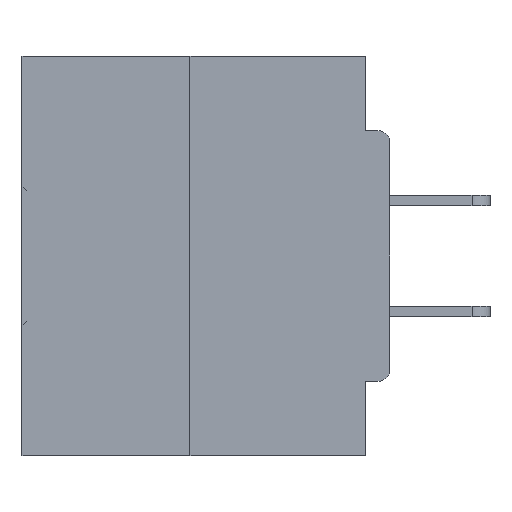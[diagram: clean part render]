
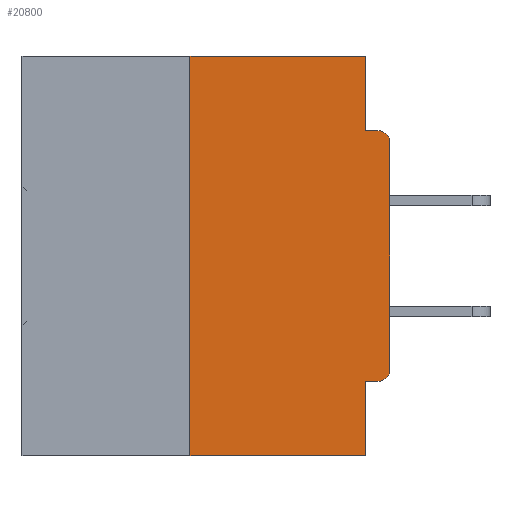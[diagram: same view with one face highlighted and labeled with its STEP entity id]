
A CAD part, left-side view. The second image highlights one B-rep face of the part: STEP entity #20800.
In plain terms, the highlighted planar face has unit normal (-1, 0, 0).
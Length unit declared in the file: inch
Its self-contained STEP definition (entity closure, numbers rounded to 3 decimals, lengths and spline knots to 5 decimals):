
#167 = VERTEX_POINT ( 'NONE', #30336 ) ;
#1050 = CARTESIAN_POINT ( 'NONE',  ( 0., 0.46, 0. ) ) ;
#2170 = VECTOR ( 'NONE', #42823, 39.37008 ) ;
#2192 = VECTOR ( 'NONE', #34902, 39.37008 ) ;
#2277 = LINE ( 'NONE', #28253, #13767 ) ;
#2855 = CARTESIAN_POINT ( 'NONE',  ( 0., 0.015, -0.0935 ) ) ;
#2877 = DIRECTION ( 'NONE',  ( -1., 0., 0. ) ) ;
#3250 = LINE ( 'NONE', #1050, #27446 ) ;
#4359 = CARTESIAN_POINT ( 'NONE',  ( 0., 0.031, 0. ) ) ;
#4479 = DIRECTION ( 'NONE',  ( 0., 0., 1. ) ) ;
#4711 = CARTESIAN_POINT ( 'NONE',  ( 0., 0.031, -0.5 ) ) ;
#4830 = AXIS2_PLACEMENT_3D ( 'NONE', #22929, #5568, #40693 ) ;
#5480 = VERTEX_POINT ( 'NONE', #2855 ) ;
#5568 = DIRECTION ( 'NONE',  ( 1., 0., 0. ) ) ;
#5937 = CARTESIAN_POINT ( 'NONE',  ( 0., 0.015, -0.3915 ) ) ;
#6063 = CARTESIAN_POINT ( 'NONE',  ( 0., 0.25, 0. ) ) ;
#6618 = CARTESIAN_POINT ( 'NONE',  ( 0., 0., -0.1085 ) ) ;
#7210 = DIRECTION ( 'NONE',  ( 0., -1., 0. ) ) ;
#8270 = EDGE_CURVE ( 'NONE', #15106, #21695, #12158, .T. ) ;
#8467 = CARTESIAN_POINT ( 'NONE',  ( 0., 0., -0.4065 ) ) ;
#8943 = EDGE_CURVE ( 'NONE', #15106, #167, #39722, .T. ) ;
#8954 = DIRECTION ( 'NONE',  ( -1., 0., 0. ) ) ;
#9755 = FACE_OUTER_BOUND ( 'NONE', #16132, .T. ) ;
#9790 = ORIENTED_EDGE ( 'NONE', *, *, #42804, .F. ) ;
#9899 = CARTESIAN_POINT ( 'NONE',  ( 0., 0.031, -0.4065 ) ) ;
#10273 = EDGE_CURVE ( 'NONE', #17444, #37389, #21950, .T. ) ;
#11295 = DIRECTION ( 'NONE',  ( 0., 0., -1. ) ) ;
#12158 = LINE ( 'NONE', #8467, #38126 ) ;
#12465 = PLANE ( 'NONE',  #4830 ) ;
#13767 = VECTOR ( 'NONE', #7210, 39.37008 ) ;
#13922 = ORIENTED_EDGE ( 'NONE', *, *, #30022, .T. ) ;
#14165 = CIRCLE ( 'NONE', #31103, 0.015 ) ;
#14408 = ORIENTED_EDGE ( 'NONE', *, *, #20055, .F. ) ;
#15106 = VERTEX_POINT ( 'NONE', #30540 ) ;
#16132 = EDGE_LOOP ( 'NONE', ( #14408, #29965, #29493, #41992, #29575, #18487, #26755, #13922, #43258, #9790 ) ) ;
#16295 = LINE ( 'NONE', #6063, #39518 ) ;
#16610 = DIRECTION ( 'NONE',  ( 0., 0., 1. ) ) ;
#17444 = VERTEX_POINT ( 'NONE', #32879 ) ;
#17700 = AXIS2_PLACEMENT_3D ( 'NONE', #5937, #2877, #38313 ) ;
#17887 = VERTEX_POINT ( 'NONE', #24301 ) ;
#18487 = ORIENTED_EDGE ( 'NONE', *, *, #8943, .T. ) ;
#18583 = EDGE_CURVE ( 'NONE', #17887, #5480, #2277, .T. ) ;
#19235 = LINE ( 'NONE', #28235, #2192 ) ;
#20055 = EDGE_CURVE ( 'NONE', #34988, #33807, #3250, .T. ) ;
#20800 = ADVANCED_FACE ( 'NONE', ( #9755 ), #12465, .F. ) ;
#21695 = VERTEX_POINT ( 'NONE', #9899 ) ;
#21950 = LINE ( 'NONE', #24924, #2170 ) ;
#22608 = EDGE_CURVE ( 'NONE', #167, #43945, #30040, .T. ) ;
#22929 = CARTESIAN_POINT ( 'NONE',  ( 0., 0.46, 0. ) ) ;
#23532 = CARTESIAN_POINT ( 'NONE',  ( 0., 0.25, 0. ) ) ;
#24166 = VECTOR ( 'NONE', #11295, 39.37008 ) ;
#24301 = CARTESIAN_POINT ( 'NONE',  ( 0., 0.031, -0.0935 ) ) ;
#24924 = CARTESIAN_POINT ( 'NONE',  ( 0., 0.46, -0.5 ) ) ;
#26755 = ORIENTED_EDGE ( 'NONE', *, *, #22608, .T. ) ;
#27446 = VECTOR ( 'NONE', #33836, 39.37008 ) ;
#28235 = CARTESIAN_POINT ( 'NONE',  ( 0., 0.031, -0.5 ) ) ;
#28253 = CARTESIAN_POINT ( 'NONE',  ( 0., 0., -0.0935 ) ) ;
#29493 = ORIENTED_EDGE ( 'NONE', *, *, #10273, .T. ) ;
#29575 = ORIENTED_EDGE ( 'NONE', *, *, #8270, .F. ) ;
#29883 = CARTESIAN_POINT ( 'NONE',  ( 0., 0.015, -0.1085 ) ) ;
#29965 = ORIENTED_EDGE ( 'NONE', *, *, #37685, .F. ) ;
#30022 = EDGE_CURVE ( 'NONE', #43945, #5480, #14165, .T. ) ;
#30040 = LINE ( 'NONE', #40351, #44885 ) ;
#30336 = CARTESIAN_POINT ( 'NONE',  ( 0., 0., -0.3915 ) ) ;
#30540 = CARTESIAN_POINT ( 'NONE',  ( 0., 0.015, -0.4065 ) ) ;
#31103 = AXIS2_PLACEMENT_3D ( 'NONE', #29883, #8954, #44315 ) ;
#32312 = CARTESIAN_POINT ( 'NONE',  ( 0., 0.031, 0. ) ) ;
#32879 = CARTESIAN_POINT ( 'NONE',  ( 0., 0.25, -0.5 ) ) ;
#33601 = LINE ( 'NONE', #32312, #24166 ) ;
#33807 = VERTEX_POINT ( 'NONE', #4359 ) ;
#33836 = DIRECTION ( 'NONE',  ( 0., -1., 0. ) ) ;
#34902 = DIRECTION ( 'NONE',  ( 0., 0., -1. ) ) ;
#34988 = VERTEX_POINT ( 'NONE', #23532 ) ;
#37389 = VERTEX_POINT ( 'NONE', #4711 ) ;
#37685 = EDGE_CURVE ( 'NONE', #17444, #34988, #16295, .T. ) ;
#38126 = VECTOR ( 'NONE', #43688, 39.37008 ) ;
#38313 = DIRECTION ( 'NONE',  ( 0., 0., -1. ) ) ;
#39518 = VECTOR ( 'NONE', #16610, 39.37008 ) ;
#39722 = CIRCLE ( 'NONE', #17700, 0.015 ) ;
#40351 = CARTESIAN_POINT ( 'NONE',  ( 0., 0., 0. ) ) ;
#40693 = DIRECTION ( 'NONE',  ( 0., 0., -1. ) ) ;
#41992 = ORIENTED_EDGE ( 'NONE', *, *, #42630, .F. ) ;
#42630 = EDGE_CURVE ( 'NONE', #21695, #37389, #19235, .T. ) ;
#42804 = EDGE_CURVE ( 'NONE', #33807, #17887, #33601, .T. ) ;
#42823 = DIRECTION ( 'NONE',  ( 0., -1., 0. ) ) ;
#43258 = ORIENTED_EDGE ( 'NONE', *, *, #18583, .F. ) ;
#43688 = DIRECTION ( 'NONE',  ( 0., 1., 0. ) ) ;
#43945 = VERTEX_POINT ( 'NONE', #6618 ) ;
#44315 = DIRECTION ( 'NONE',  ( 0., 0., -1. ) ) ;
#44885 = VECTOR ( 'NONE', #4479, 39.37008 ) ;
